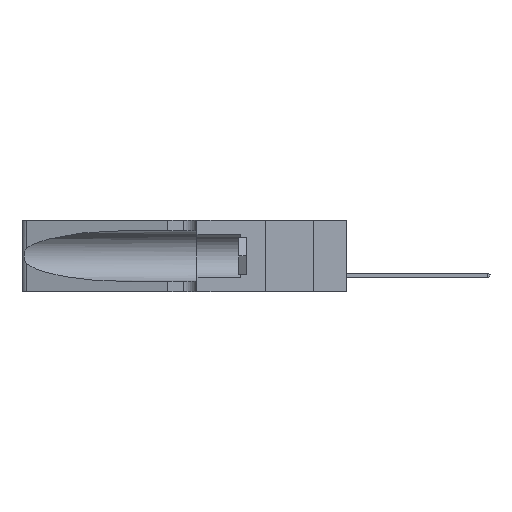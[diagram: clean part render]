
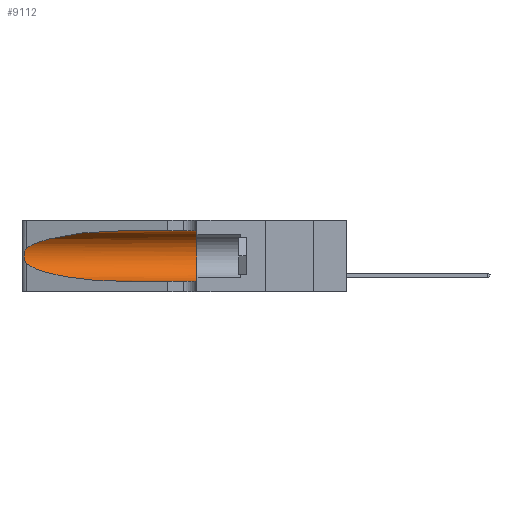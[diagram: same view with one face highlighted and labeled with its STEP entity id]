
A CAD part, left-side view. The second image highlights one B-rep face of the part: STEP entity #9112.
In plain terms, the highlighted cylindrical face has radius 3.308 mm (diameter 6.617 mm), a partial arc.
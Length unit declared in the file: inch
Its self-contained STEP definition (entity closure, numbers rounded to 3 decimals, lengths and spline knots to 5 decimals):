
#734 = CARTESIAN_POINT ( 'NONE',  ( 0.1305, 1.61858, 0.185 ) ) ;
#1076 = VECTOR ( 'NONE', #31358, 39.37008 ) ;
#1268 = VECTOR ( 'NONE', #19116, 39.37008 ) ;
#2463 = CARTESIAN_POINT ( 'NONE',  ( 0.1305, 0.35, 0.05475 ) ) ;
#2741 = CIRCLE ( 'NONE', #36507, 0.13025 ) ;
#3667 = EDGE_CURVE ( 'NONE', #33737, #8285, #18657, .T. ) ;
#5499 = CARTESIAN_POINT ( 'NONE',  ( 0.26075, 1.23896, 0.19203 ) ) ;
#5598 = CARTESIAN_POINT ( 'NONE',  ( 0.18966, 0.96281, 0.31525 ) ) ;
#5649 = CARTESIAN_POINT ( 'NONE',  ( 0.25789, 1.23486, 0.15765 ) ) ;
#6162 = ORIENTED_EDGE ( 'NONE', *, *, #19732, .T. ) ;
#8285 = VERTEX_POINT ( 'NONE', #33772 ) ;
#8998 = LINE ( 'NONE', #26498, #1268 ) ;
#9112 = ADVANCED_FACE ( 'NONE', ( #14564 ), #11519, .F. ) ;
#10038 = EDGE_CURVE ( 'NONE', #37251, #33511, #8998, .T. ) ;
#11338 = CARTESIAN_POINT ( 'NONE',  ( 0.1305, 0.72297, 0.05475 ) ) ;
#11519 = CYLINDRICAL_SURFACE ( 'NONE', #26442, 0.13025 ) ;
#11731 = CARTESIAN_POINT ( 'NONE',  ( 0.2373, 1.15595, 0.28018 ) ) ;
#12333 = ORIENTED_EDGE ( 'NONE', *, *, #15194, .T. ) ;
#13651 = DIRECTION ( 'NONE',  ( 0., -1., 0. ) ) ;
#14564 = FACE_OUTER_BOUND ( 'NONE', #19006, .T. ) ;
#14905 = CARTESIAN_POINT ( 'NONE',  ( 0.25487, 1.22718, 0.14631 ) ) ;
#15194 = EDGE_CURVE ( 'NONE', #35573, #33737, #27501, .T. ) ;
#15419 = CARTESIAN_POINT ( 'NONE',  ( 0.25856, 1.23593, 0.16098 ) ) ;
#15710 = CARTESIAN_POINT ( 'NONE',  ( 0.25854, 1.2359, 0.20912 ) ) ;
#17935 = EDGE_CURVE ( 'NONE', #33511, #39066, #2741, .T. ) ;
#18090 = CARTESIAN_POINT ( 'NONE',  ( 0.2373, 1.15595, 0.08982 ) ) ;
#18533 = CARTESIAN_POINT ( 'NONE',  ( 0.25555, 1.22994, 0.2215 ) ) ;
#18657 =( BOUNDED_CURVE ( )  B_SPLINE_CURVE ( 3, ( #39702, #18090, #21350, #11338 ),
 .UNSPECIFIED., .F., .T. ) 
 B_SPLINE_CURVE_WITH_KNOTS ( ( 4, 4 ),
 ( 3.44316, 4.71239 ),
 .UNSPECIFIED. ) 
 CURVE ( )  GEOMETRIC_REPRESENTATION_ITEM ( )  RATIONAL_B_SPLINE_CURVE ( ( 1., 0.87, 0.87, 1. ) ) 
 REPRESENTATION_ITEM ( '' )  );
#18679 = CARTESIAN_POINT ( 'NONE',  ( 0.25487, 1.22718, 0.22369 ) ) ;
#19006 = EDGE_LOOP ( 'NONE', ( #6162, #12333, #22481, #31481, #30459, #31056 ) ) ;
#19116 = DIRECTION ( 'NONE',  ( 0., -1., 0. ) ) ;
#19394 = DIRECTION ( 'NONE',  ( 0., 0., 1. ) ) ;
#19732 = EDGE_CURVE ( 'NONE', #37251, #35573, #31906, .T. ) ;
#19780 = DIRECTION ( 'NONE',  ( 0., 1., 0. ) ) ;
#21350 = CARTESIAN_POINT ( 'NONE',  ( 0.18966, 0.96281, 0.05475 ) ) ;
#21609 = CARTESIAN_POINT ( 'NONE',  ( 0.25487, 1.22718, 0.22369 ) ) ;
#21944 = CARTESIAN_POINT ( 'NONE',  ( 0.25487, 1.22718, 0.14631 ) ) ;
#22481 = ORIENTED_EDGE ( 'NONE', *, *, #3667, .T. ) ;
#23609 = DIRECTION ( 'NONE',  ( 0., 0., -1. ) ) ;
#25095 = CARTESIAN_POINT ( 'NONE',  ( 0.26075, 1.23896, 0.178 ) ) ;
#25177 = CARTESIAN_POINT ( 'NONE',  ( 0.1305, 1.61858, 0.05475 ) ) ;
#25232 = CARTESIAN_POINT ( 'NONE',  ( 0.25639, 1.23184, 0.21858 ) ) ;
#26442 = AXIS2_PLACEMENT_3D ( 'NONE', #734, #13651, #23609 ) ;
#26498 = CARTESIAN_POINT ( 'NONE',  ( 0.1305, 1.61858, 0.31525 ) ) ;
#27501 = B_SPLINE_CURVE_WITH_KNOTS ( 'NONE', 3,
 ( #18679, #18533, #25232, #28072, #15710, #31852, #5499, #25095, #31566, #15419, #5649, #38211, #41295, #21944 ),
 .UNSPECIFIED., .F., .F.,
 ( 4, 2, 2, 2, 2, 2, 4 ),
 ( 0., 0.00027, 0.00053, 0.00107, 0.0016, 0.00187, 0.00214 ),
 .UNSPECIFIED. ) ;
#28072 = CARTESIAN_POINT ( 'NONE',  ( 0.25787, 1.23484, 0.2124 ) ) ;
#30459 = ORIENTED_EDGE ( 'NONE', *, *, #17935, .F. ) ;
#31056 = ORIENTED_EDGE ( 'NONE', *, *, #10038, .F. ) ;
#31358 = DIRECTION ( 'NONE',  ( 0., -1., 0. ) ) ;
#31481 = ORIENTED_EDGE ( 'NONE', *, *, #36445, .T. ) ;
#31566 = CARTESIAN_POINT ( 'NONE',  ( 0.26017, 1.23833, 0.17102 ) ) ;
#31852 = CARTESIAN_POINT ( 'NONE',  ( 0.26018, 1.23835, 0.19895 ) ) ;
#31906 =( BOUNDED_CURVE ( )  B_SPLINE_CURVE ( 3, ( #40947, #5598, #11731, #21609 ),
 .UNSPECIFIED., .F., .T. ) 
 B_SPLINE_CURVE_WITH_KNOTS ( ( 4, 4 ),
 ( 1.5708, 2.84003 ),
 .UNSPECIFIED. ) 
 CURVE ( )  GEOMETRIC_REPRESENTATION_ITEM ( )  RATIONAL_B_SPLINE_CURVE ( ( 1., 0.87, 0.87, 1. ) ) 
 REPRESENTATION_ITEM ( '' )  );
#32295 = CARTESIAN_POINT ( 'NONE',  ( 0.1305, 0.72297, 0.31525 ) ) ;
#33511 = VERTEX_POINT ( 'NONE', #33557 ) ;
#33557 = CARTESIAN_POINT ( 'NONE',  ( 0.1305, 0.35, 0.31525 ) ) ;
#33737 = VERTEX_POINT ( 'NONE', #14905 ) ;
#33772 = CARTESIAN_POINT ( 'NONE',  ( 0.1305, 0.72297, 0.05475 ) ) ;
#35573 = VERTEX_POINT ( 'NONE', #39147 ) ;
#36445 = EDGE_CURVE ( 'NONE', #8285, #39066, #40641, .T. ) ;
#36507 = AXIS2_PLACEMENT_3D ( 'NONE', #38780, #19780, #19394 ) ;
#37251 = VERTEX_POINT ( 'NONE', #32295 ) ;
#38211 = CARTESIAN_POINT ( 'NONE',  ( 0.25639, 1.23186, 0.15144 ) ) ;
#38780 = CARTESIAN_POINT ( 'NONE',  ( 0.1305, 0.35, 0.185 ) ) ;
#39066 = VERTEX_POINT ( 'NONE', #2463 ) ;
#39147 = CARTESIAN_POINT ( 'NONE',  ( 0.25487, 1.22718, 0.22369 ) ) ;
#39702 = CARTESIAN_POINT ( 'NONE',  ( 0.25487, 1.22718, 0.14631 ) ) ;
#40641 = LINE ( 'NONE', #25177, #1076 ) ;
#40947 = CARTESIAN_POINT ( 'NONE',  ( 0.1305, 0.72297, 0.31525 ) ) ;
#41295 = CARTESIAN_POINT ( 'NONE',  ( 0.25555, 1.22993, 0.14849 ) ) ;
